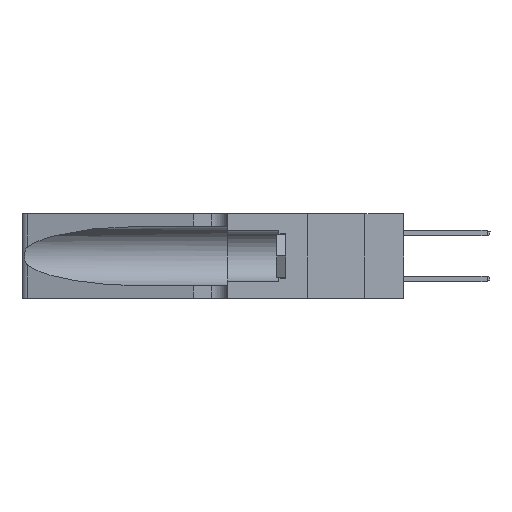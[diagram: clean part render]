
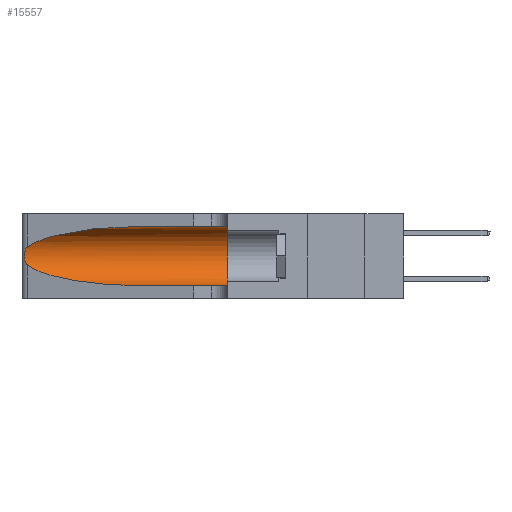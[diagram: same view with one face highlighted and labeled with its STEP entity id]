
A CAD part, left-side view. The second image highlights one B-rep face of the part: STEP entity #15557.
In plain terms, the highlighted cylindrical face has radius 3.308 mm (diameter 6.617 mm), a partial arc.
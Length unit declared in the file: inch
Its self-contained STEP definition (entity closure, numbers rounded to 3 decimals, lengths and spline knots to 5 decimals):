
#968 = CARTESIAN_POINT ( 'NONE',  ( 0.25789, 1.23486, 0.15765 ) ) ;
#1163 = VERTEX_POINT ( 'NONE', #5758 ) ;
#1444 = EDGE_CURVE ( 'NONE', #35244, #3756, #15011, .T. ) ;
#3226 = EDGE_CURVE ( 'NONE', #13084, #35244, #15963, .T. ) ;
#3756 = VERTEX_POINT ( 'NONE', #4092 ) ;
#4092 = CARTESIAN_POINT ( 'NONE',  ( 0.1305, 0.35, 0.05475 ) ) ;
#4180 = CARTESIAN_POINT ( 'NONE',  ( 0.25555, 1.22993, 0.14849 ) ) ;
#4280 = ORIENTED_EDGE ( 'NONE', *, *, #18545, .T. ) ;
#5613 = LINE ( 'NONE', #35656, #13992 ) ;
#5758 = CARTESIAN_POINT ( 'NONE',  ( 0.25487, 1.22718, 0.22369 ) ) ;
#5813 = CARTESIAN_POINT ( 'NONE',  ( 0.1305, 0.35, 0.185 ) ) ;
#5963 = CIRCLE ( 'NONE', #32902, 0.13025 ) ;
#7171 = CYLINDRICAL_SURFACE ( 'NONE', #23135, 0.13025 ) ;
#7215 = CARTESIAN_POINT ( 'NONE',  ( 0.25555, 1.22994, 0.2215 ) ) ;
#8558 = CARTESIAN_POINT ( 'NONE',  ( 0.1305, 0.72297, 0.31525 ) ) ;
#8981 = DIRECTION ( 'NONE',  ( 0., 0., 1. ) ) ;
#9373 = VERTEX_POINT ( 'NONE', #35193 ) ;
#10397 = CARTESIAN_POINT ( 'NONE',  ( 0.25787, 1.23484, 0.2124 ) ) ;
#10714 = EDGE_CURVE ( 'NONE', #12819, #9373, #5613, .T. ) ;
#10950 = CARTESIAN_POINT ( 'NONE',  ( 0.1305, 0.72297, 0.31525 ) ) ;
#12102 = CARTESIAN_POINT ( 'NONE',  ( 0.2373, 1.15595, 0.08982 ) ) ;
#12271 = EDGE_CURVE ( 'NONE', #9373, #3756, #5963, .T. ) ;
#12819 = VERTEX_POINT ( 'NONE', #8558 ) ;
#13084 = VERTEX_POINT ( 'NONE', #16122 ) ;
#13108 = ORIENTED_EDGE ( 'NONE', *, *, #3226, .T. ) ;
#13561 = CARTESIAN_POINT ( 'NONE',  ( 0.26018, 1.23835, 0.19895 ) ) ;
#13992 = VECTOR ( 'NONE', #23216, 39.37008 ) ;
#14618 = CARTESIAN_POINT ( 'NONE',  ( 0.1305, 0.72297, 0.05475 ) ) ;
#15011 = LINE ( 'NONE', #16490, #29597 ) ;
#15268 = CARTESIAN_POINT ( 'NONE',  ( 0.1305, 0.72297, 0.05475 ) ) ;
#15557 = ADVANCED_FACE ( 'NONE', ( #23858 ), #7171, .F. ) ;
#15814 = DIRECTION ( 'NONE',  ( 0., -1., 0. ) ) ;
#15963 =( BOUNDED_CURVE ( )  B_SPLINE_CURVE ( 3, ( #30609, #12102, #33860, #15268 ),
 .UNSPECIFIED., .F., .F. ) 
 B_SPLINE_CURVE_WITH_KNOTS ( ( 4, 4 ),
 ( 3.44316, 4.71239 ),
 .UNSPECIFIED. ) 
 CURVE ( )  GEOMETRIC_REPRESENTATION_ITEM ( )  RATIONAL_B_SPLINE_CURVE ( ( 1., 0.87, 0.87, 1. ) ) 
 REPRESENTATION_ITEM ( '' )  );
#16060 = ORIENTED_EDGE ( 'NONE', *, *, #12271, .F. ) ;
#16122 = CARTESIAN_POINT ( 'NONE',  ( 0.25487, 1.22718, 0.14631 ) ) ;
#16490 = CARTESIAN_POINT ( 'NONE',  ( 0.1305, 1.61858, 0.05475 ) ) ;
#16721 = CARTESIAN_POINT ( 'NONE',  ( 0.26075, 1.23896, 0.178 ) ) ;
#17289 = CARTESIAN_POINT ( 'NONE',  ( 0.2373, 1.15595, 0.28018 ) ) ;
#18054 = ORIENTED_EDGE ( 'NONE', *, *, #10714, .F. ) ;
#18545 = EDGE_CURVE ( 'NONE', #12819, #1163, #20242, .T. ) ;
#18985 = CARTESIAN_POINT ( 'NONE',  ( 0.1305, 1.61858, 0.185 ) ) ;
#19883 = CARTESIAN_POINT ( 'NONE',  ( 0.25856, 1.23593, 0.16098 ) ) ;
#20242 =( BOUNDED_CURVE ( )  B_SPLINE_CURVE ( 3, ( #10950, #35850, #17289, #38962 ),
 .UNSPECIFIED., .F., .F. ) 
 B_SPLINE_CURVE_WITH_KNOTS ( ( 4, 4 ),
 ( 1.5708, 2.84003 ),
 .UNSPECIFIED. ) 
 CURVE ( )  GEOMETRIC_REPRESENTATION_ITEM ( )  RATIONAL_B_SPLINE_CURVE ( ( 1., 0.87, 0.87, 1. ) ) 
 REPRESENTATION_ITEM ( '' )  );
#22634 = DIRECTION ( 'NONE',  ( 0., -1., 0. ) ) ;
#22992 = CARTESIAN_POINT ( 'NONE',  ( 0.25639, 1.23186, 0.15144 ) ) ;
#23135 = AXIS2_PLACEMENT_3D ( 'NONE', #18985, #15814, #37388 ) ;
#23216 = DIRECTION ( 'NONE',  ( 0., -1., 0. ) ) ;
#23385 = ORIENTED_EDGE ( 'NONE', *, *, #1444, .T. ) ;
#23858 = FACE_OUTER_BOUND ( 'NONE', #28394, .T. ) ;
#24456 = B_SPLINE_CURVE_WITH_KNOTS ( 'NONE', 3,
 ( #38291, #7215, #29085, #10397, #32184, #13561, #35291, #16721, #38435, #19883, #968, #22992, #4180, #26117 ),
 .UNSPECIFIED., .F., .F.,
 ( 4, 2, 2, 2, 2, 2, 4 ),
 ( 0., 0.00027, 0.00053, 0.00107, 0.0016, 0.00187, 0.00214 ),
 .UNSPECIFIED. ) ;
#26117 = CARTESIAN_POINT ( 'NONE',  ( 0.25487, 1.22718, 0.14631 ) ) ;
#27720 = DIRECTION ( 'NONE',  ( 0., 1., 0. ) ) ;
#28394 = EDGE_LOOP ( 'NONE', ( #4280, #28704, #13108, #23385, #16060, #18054 ) ) ;
#28704 = ORIENTED_EDGE ( 'NONE', *, *, #37602, .T. ) ;
#29085 = CARTESIAN_POINT ( 'NONE',  ( 0.25639, 1.23184, 0.21858 ) ) ;
#29597 = VECTOR ( 'NONE', #22634, 39.37008 ) ;
#30609 = CARTESIAN_POINT ( 'NONE',  ( 0.25487, 1.22718, 0.14631 ) ) ;
#32184 = CARTESIAN_POINT ( 'NONE',  ( 0.25854, 1.2359, 0.20912 ) ) ;
#32902 = AXIS2_PLACEMENT_3D ( 'NONE', #5813, #27720, #8981 ) ;
#33860 = CARTESIAN_POINT ( 'NONE',  ( 0.18966, 0.96281, 0.05475 ) ) ;
#35193 = CARTESIAN_POINT ( 'NONE',  ( 0.1305, 0.35, 0.31525 ) ) ;
#35244 = VERTEX_POINT ( 'NONE', #14618 ) ;
#35291 = CARTESIAN_POINT ( 'NONE',  ( 0.26075, 1.23896, 0.19203 ) ) ;
#35656 = CARTESIAN_POINT ( 'NONE',  ( 0.1305, 1.61858, 0.31525 ) ) ;
#35850 = CARTESIAN_POINT ( 'NONE',  ( 0.18966, 0.96281, 0.31525 ) ) ;
#37388 = DIRECTION ( 'NONE',  ( 0., 0., -1. ) ) ;
#37602 = EDGE_CURVE ( 'NONE', #1163, #13084, #24456, .T. ) ;
#38291 = CARTESIAN_POINT ( 'NONE',  ( 0.25487, 1.22718, 0.22369 ) ) ;
#38435 = CARTESIAN_POINT ( 'NONE',  ( 0.26017, 1.23833, 0.17102 ) ) ;
#38962 = CARTESIAN_POINT ( 'NONE',  ( 0.25487, 1.22718, 0.22369 ) ) ;
